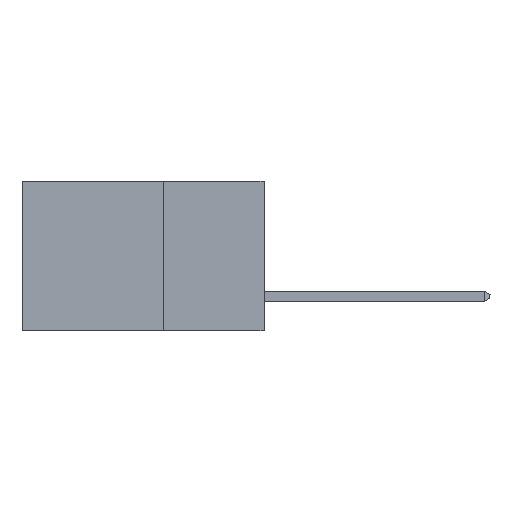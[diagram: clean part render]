
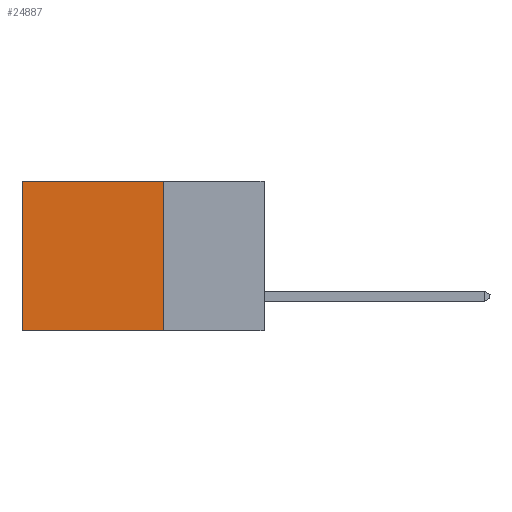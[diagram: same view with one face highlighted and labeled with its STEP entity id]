
A CAD part, left-side view. The second image highlights one B-rep face of the part: STEP entity #24887.
In plain terms, the highlighted planar face has unit normal (-1, 0, 0).
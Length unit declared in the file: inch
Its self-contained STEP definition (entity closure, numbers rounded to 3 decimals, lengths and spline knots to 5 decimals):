
#161 = CARTESIAN_POINT ( 'NONE',  ( 0.2615, 0.25, 0. ) ) ;
#467 = CARTESIAN_POINT ( 'NONE',  ( 0.2615, 0.25, -0.37 ) ) ;
#872 = CARTESIAN_POINT ( 'NONE',  ( 0.2615, 0.6, -0.37 ) ) ;
#1141 = FACE_OUTER_BOUND ( 'NONE', #12668, .T. ) ;
#1221 = ORIENTED_EDGE ( 'NONE', *, *, #8212, .F. ) ;
#1266 = DIRECTION ( 'NONE',  ( 0., 0., -1. ) ) ;
#3201 = DIRECTION ( 'NONE',  ( 1., 0., 0. ) ) ;
#3550 = AXIS2_PLACEMENT_3D ( 'NONE', #16712, #3201, #1266 ) ;
#3827 = DIRECTION ( 'NONE',  ( 0., 0., -1. ) ) ;
#4696 = VECTOR ( 'NONE', #20629, 39.37008 ) ;
#6165 = LINE ( 'NONE', #20183, #21048 ) ;
#7648 = EDGE_CURVE ( 'NONE', #19786, #9389, #6165, .T. ) ;
#8115 = VERTEX_POINT ( 'NONE', #467 ) ;
#8212 = EDGE_CURVE ( 'NONE', #8115, #9389, #21004, .T. ) ;
#8951 = PLANE ( 'NONE',  #3550 ) ;
#9389 = VERTEX_POINT ( 'NONE', #872 ) ;
#10809 = CARTESIAN_POINT ( 'NONE',  ( 0.2615, 0.25, -0.37 ) ) ;
#11676 = DIRECTION ( 'NONE',  ( 0., 1., 0. ) ) ;
#11908 = DIRECTION ( 'NONE',  ( 0., 0., -1. ) ) ;
#12668 = EDGE_LOOP ( 'NONE', ( #16453, #1221, #20761, #17261 ) ) ;
#13233 = VECTOR ( 'NONE', #3827, 39.37008 ) ;
#14789 = CARTESIAN_POINT ( 'NONE',  ( 0.2615, 0.25, 0. ) ) ;
#15621 = LINE ( 'NONE', #161, #21432 ) ;
#16453 = ORIENTED_EDGE ( 'NONE', *, *, #7648, .T. ) ;
#16708 = CARTESIAN_POINT ( 'NONE',  ( 0.2615, 0.6, 0. ) ) ;
#16712 = CARTESIAN_POINT ( 'NONE',  ( 0.2615, 0.25, -0.37 ) ) ;
#17261 = ORIENTED_EDGE ( 'NONE', *, *, #21213, .T. ) ;
#18652 = VERTEX_POINT ( 'NONE', #14789 ) ;
#19537 = EDGE_CURVE ( 'NONE', #18652, #8115, #20947, .T. ) ;
#19786 = VERTEX_POINT ( 'NONE', #16708 ) ;
#20183 = CARTESIAN_POINT ( 'NONE',  ( 0.2615, 0.6, -0.37 ) ) ;
#20629 = DIRECTION ( 'NONE',  ( 0., 1., 0. ) ) ;
#20761 = ORIENTED_EDGE ( 'NONE', *, *, #19537, .F. ) ;
#20947 = LINE ( 'NONE', #23096, #13233 ) ;
#21004 = LINE ( 'NONE', #10809, #4696 ) ;
#21048 = VECTOR ( 'NONE', #11908, 39.37008 ) ;
#21213 = EDGE_CURVE ( 'NONE', #18652, #19786, #15621, .T. ) ;
#21432 = VECTOR ( 'NONE', #11676, 39.37008 ) ;
#23096 = CARTESIAN_POINT ( 'NONE',  ( 0.2615, 0.25, -0.37 ) ) ;
#24887 = ADVANCED_FACE ( 'NONE', ( #1141 ), #8951, .F. ) ;
